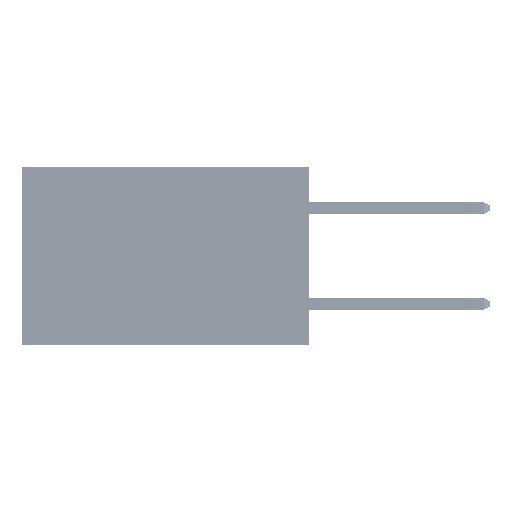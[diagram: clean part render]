
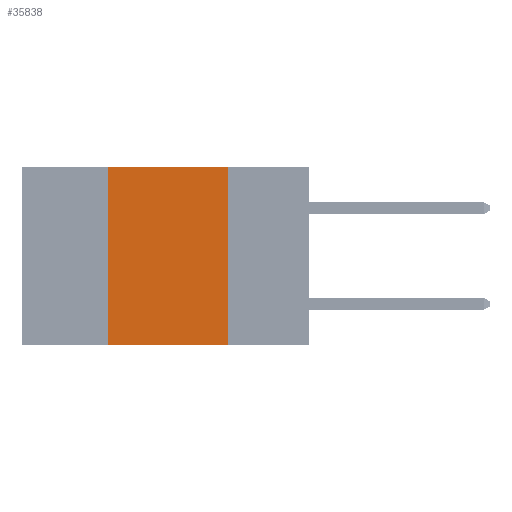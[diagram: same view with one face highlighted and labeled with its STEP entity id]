
A CAD part, left-side view. The second image highlights one B-rep face of the part: STEP entity #35838.
In plain terms, the highlighted planar face has unit normal (-1, 0, 0).
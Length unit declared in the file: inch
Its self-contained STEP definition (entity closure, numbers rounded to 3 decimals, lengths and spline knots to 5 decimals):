
#651 = CARTESIAN_POINT ( 'NONE',  ( 0., 0.6, 0. ) ) ;
#1007 = PLANE ( 'NONE',  #15834 ) ;
#4437 = EDGE_CURVE ( 'NONE', #34201, #35896, #27908, .T. ) ;
#4678 = DIRECTION ( 'NONE',  ( 0., -1., 0. ) ) ;
#6168 = VERTEX_POINT ( 'NONE', #12808 ) ;
#6556 = FACE_OUTER_BOUND ( 'NONE', #42314, .T. ) ;
#6931 = EDGE_CURVE ( 'NONE', #6168, #46921, #7340, .T. ) ;
#7340 = LINE ( 'NONE', #28941, #38866 ) ;
#12471 = CARTESIAN_POINT ( 'NONE',  ( 0., 0.17, -0.37 ) ) ;
#12808 = CARTESIAN_POINT ( 'NONE',  ( 0., 0.42, 0. ) ) ;
#15080 = EDGE_CURVE ( 'NONE', #34201, #6168, #44875, .T. ) ;
#15834 = AXIS2_PLACEMENT_3D ( 'NONE', #651, #25606, #29718 ) ;
#16305 = CARTESIAN_POINT ( 'NONE',  ( 0., 0.17, 0. ) ) ;
#17219 = ORIENTED_EDGE ( 'NONE', *, *, #4437, .T. ) ;
#17758 = DIRECTION ( 'NONE',  ( 0., 0., -1. ) ) ;
#19271 = CARTESIAN_POINT ( 'NONE',  ( 0., 0.42, 0. ) ) ;
#19834 = DIRECTION ( 'NONE',  ( 0., -1., 0. ) ) ;
#21472 = VECTOR ( 'NONE', #19834, 39.37008 ) ;
#25606 = DIRECTION ( 'NONE',  ( 1., 0., 0. ) ) ;
#27908 = LINE ( 'NONE', #52475, #21472 ) ;
#28288 = EDGE_CURVE ( 'NONE', #46921, #35896, #39821, .T. ) ;
#28941 = CARTESIAN_POINT ( 'NONE',  ( 0., 0.6, 0. ) ) ;
#29718 = DIRECTION ( 'NONE',  ( 0., 0., -1. ) ) ;
#32669 = VECTOR ( 'NONE', #39891, 39.37008 ) ;
#32732 = ORIENTED_EDGE ( 'NONE', *, *, #6931, .F. ) ;
#34201 = VERTEX_POINT ( 'NONE', #38175 ) ;
#35838 = ADVANCED_FACE ( 'NONE', ( #6556 ), #1007, .F. ) ;
#35896 = VERTEX_POINT ( 'NONE', #12471 ) ;
#35948 = VECTOR ( 'NONE', #17758, 39.37008 ) ;
#37344 = ORIENTED_EDGE ( 'NONE', *, *, #15080, .F. ) ;
#38175 = CARTESIAN_POINT ( 'NONE',  ( 0., 0.42, -0.37 ) ) ;
#38866 = VECTOR ( 'NONE', #4678, 39.37008 ) ;
#39821 = LINE ( 'NONE', #41985, #35948 ) ;
#39891 = DIRECTION ( 'NONE',  ( 0., 0., 1. ) ) ;
#41707 = ORIENTED_EDGE ( 'NONE', *, *, #28288, .F. ) ;
#41985 = CARTESIAN_POINT ( 'NONE',  ( 0., 0.17, 0. ) ) ;
#42314 = EDGE_LOOP ( 'NONE', ( #41707, #32732, #37344, #17219 ) ) ;
#44875 = LINE ( 'NONE', #19271, #32669 ) ;
#46921 = VERTEX_POINT ( 'NONE', #16305 ) ;
#52475 = CARTESIAN_POINT ( 'NONE',  ( 0., 0.6, -0.37 ) ) ;
